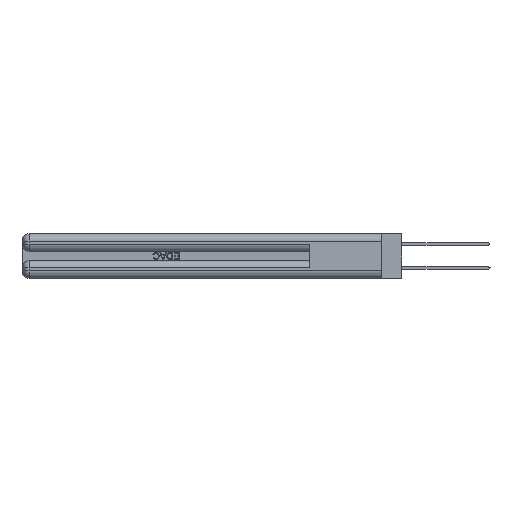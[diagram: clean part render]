
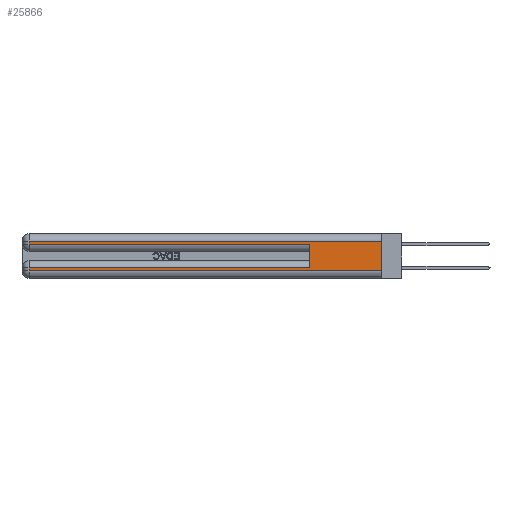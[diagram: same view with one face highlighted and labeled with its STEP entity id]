
A CAD part, left-side view. The second image highlights one B-rep face of the part: STEP entity #25866.
In plain terms, the highlighted planar face has unit normal (-1, 0, 0).
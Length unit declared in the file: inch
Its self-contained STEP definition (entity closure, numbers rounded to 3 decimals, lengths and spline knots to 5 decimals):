
#92 = DIRECTION ( 'NONE',  ( 0., -1., 0. ) ) ;
#1254 = EDGE_CURVE ( 'NONE', #24617, #43516, #19529, .T. ) ;
#2156 = LINE ( 'NONE', #16699, #29848 ) ;
#2284 = CARTESIAN_POINT ( 'NONE',  ( 0., 2.94, 0.085 ) ) ;
#2750 = VECTOR ( 'NONE', #37645, 39.37008 ) ;
#4744 = VECTOR ( 'NONE', #44942, 39.37008 ) ;
#4845 = CARTESIAN_POINT ( 'NONE',  ( 0., 0., 0.31 ) ) ;
#4972 = ORIENTED_EDGE ( 'NONE', *, *, #10195, .T. ) ;
#4973 = CARTESIAN_POINT ( 'NONE',  ( 0., 2.94, 0.06 ) ) ;
#5294 = VERTEX_POINT ( 'NONE', #9909 ) ;
#8114 = ORIENTED_EDGE ( 'NONE', *, *, #1254, .F. ) ;
#9450 = VERTEX_POINT ( 'NONE', #4973 ) ;
#9842 = CARTESIAN_POINT ( 'NONE',  ( 0., 2.94, 0.285 ) ) ;
#9909 = CARTESIAN_POINT ( 'NONE',  ( 0., 0., 0.31 ) ) ;
#9946 = VECTOR ( 'NONE', #31448, 39.37008 ) ;
#10195 = EDGE_CURVE ( 'NONE', #9450, #41006, #34776, .T. ) ;
#10352 = ORIENTED_EDGE ( 'NONE', *, *, #38731, .F. ) ;
#10982 = LINE ( 'NONE', #43368, #29019 ) ;
#11900 = EDGE_CURVE ( 'NONE', #30744, #43516, #10982, .T. ) ;
#12394 = LINE ( 'NONE', #30415, #2750 ) ;
#12551 = FACE_OUTER_BOUND ( 'NONE', #40293, .T. ) ;
#13666 = LINE ( 'NONE', #4845, #31695 ) ;
#14364 = LINE ( 'NONE', #41506, #4744 ) ;
#14682 = ORIENTED_EDGE ( 'NONE', *, *, #11900, .T. ) ;
#15130 = EDGE_CURVE ( 'NONE', #27122, #30744, #2156, .T. ) ;
#16619 = PLANE ( 'NONE',  #27429 ) ;
#16699 = CARTESIAN_POINT ( 'NONE',  ( 0., 2.94, 0.37 ) ) ;
#16719 = VECTOR ( 'NONE', #45567, 39.37008 ) ;
#16726 = EDGE_CURVE ( 'NONE', #29498, #9450, #31997, .T. ) ;
#18255 = EDGE_CURVE ( 'NONE', #24617, #29498, #14364, .T. ) ;
#19529 = LINE ( 'NONE', #38522, #9946 ) ;
#19975 = EDGE_CURVE ( 'NONE', #5294, #27122, #13666, .T. ) ;
#20270 = CARTESIAN_POINT ( 'NONE',  ( 0., 0., 0.37 ) ) ;
#22836 = ORIENTED_EDGE ( 'NONE', *, *, #18255, .T. ) ;
#23862 = DIRECTION ( 'NONE',  ( 0., 0., -1. ) ) ;
#24617 = VERTEX_POINT ( 'NONE', #40984 ) ;
#24916 = CARTESIAN_POINT ( 'NONE',  ( 0., 2.94, 0.37 ) ) ;
#25866 = ADVANCED_FACE ( 'NONE', ( #12551 ), #16619, .F. ) ;
#26146 = CARTESIAN_POINT ( 'NONE',  ( 0., 0.6, 0.285 ) ) ;
#26952 = ORIENTED_EDGE ( 'NONE', *, *, #15130, .T. ) ;
#27122 = VERTEX_POINT ( 'NONE', #35427 ) ;
#27429 = AXIS2_PLACEMENT_3D ( 'NONE', #20270, #45439, #23862 ) ;
#29019 = VECTOR ( 'NONE', #92, 39.37008 ) ;
#29498 = VERTEX_POINT ( 'NONE', #2284 ) ;
#29732 = VECTOR ( 'NONE', #39563, 39.37008 ) ;
#29848 = VECTOR ( 'NONE', #34992, 39.37008 ) ;
#30415 = CARTESIAN_POINT ( 'NONE',  ( 0., 0., 0.37 ) ) ;
#30744 = VERTEX_POINT ( 'NONE', #9842 ) ;
#31448 = DIRECTION ( 'NONE',  ( 0., 0., 1. ) ) ;
#31695 = VECTOR ( 'NONE', #37168, 39.37008 ) ;
#31997 = LINE ( 'NONE', #24916, #29732 ) ;
#34776 = LINE ( 'NONE', #42114, #16719 ) ;
#34992 = DIRECTION ( 'NONE',  ( 0., 0., -1. ) ) ;
#35427 = CARTESIAN_POINT ( 'NONE',  ( 0., 2.94, 0.31 ) ) ;
#37168 = DIRECTION ( 'NONE',  ( 0., 1., 0. ) ) ;
#37645 = DIRECTION ( 'NONE',  ( 0., 0., -1. ) ) ;
#38522 = CARTESIAN_POINT ( 'NONE',  ( 0., 0.6, 0.145 ) ) ;
#38731 = EDGE_CURVE ( 'NONE', #5294, #41006, #12394, .T. ) ;
#39563 = DIRECTION ( 'NONE',  ( 0., 0., -1. ) ) ;
#40293 = EDGE_LOOP ( 'NONE', ( #10352, #45473, #26952, #14682, #8114, #22836, #44783, #4972 ) ) ;
#40984 = CARTESIAN_POINT ( 'NONE',  ( 0., 0.6, 0.085 ) ) ;
#41006 = VERTEX_POINT ( 'NONE', #42982 ) ;
#41506 = CARTESIAN_POINT ( 'NONE',  ( 0., 0., 0.085 ) ) ;
#42114 = CARTESIAN_POINT ( 'NONE',  ( 0., 0., 0.06 ) ) ;
#42982 = CARTESIAN_POINT ( 'NONE',  ( 0., 0., 0.06 ) ) ;
#43368 = CARTESIAN_POINT ( 'NONE',  ( 0., 0., 0.285 ) ) ;
#43516 = VERTEX_POINT ( 'NONE', #26146 ) ;
#44783 = ORIENTED_EDGE ( 'NONE', *, *, #16726, .T. ) ;
#44942 = DIRECTION ( 'NONE',  ( 0., 1., 0. ) ) ;
#45439 = DIRECTION ( 'NONE',  ( 1., 0., 0. ) ) ;
#45473 = ORIENTED_EDGE ( 'NONE', *, *, #19975, .T. ) ;
#45567 = DIRECTION ( 'NONE',  ( 0., -1., 0. ) ) ;
